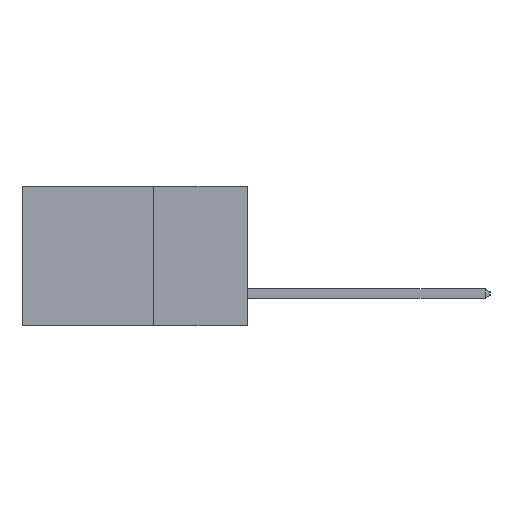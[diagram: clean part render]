
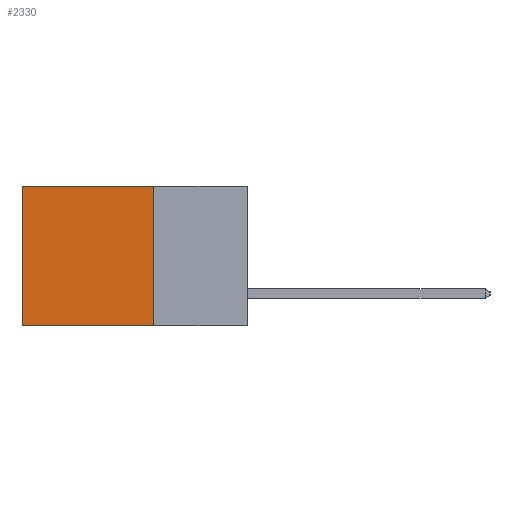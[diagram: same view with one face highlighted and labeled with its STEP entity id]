
A CAD part, left-side view. The second image highlights one B-rep face of the part: STEP entity #2330.
In plain terms, the highlighted planar face has unit normal (-1, 0, 0).
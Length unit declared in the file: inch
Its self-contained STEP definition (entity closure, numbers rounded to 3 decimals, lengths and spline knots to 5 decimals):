
#1316 = LINE ( 'NONE', #23785, #10888 ) ;
#2330 = ADVANCED_FACE ( 'NONE', ( #11259 ), #9148, .F. ) ;
#3410 = LINE ( 'NONE', #6248, #17305 ) ;
#4028 = CARTESIAN_POINT ( 'NONE',  ( 0.2615, 0.6, -0.37 ) ) ;
#4083 = DIRECTION ( 'NONE',  ( 0., 0., -1. ) ) ;
#4328 = VERTEX_POINT ( 'NONE', #19740 ) ;
#4990 = VERTEX_POINT ( 'NONE', #23582 ) ;
#5461 = VERTEX_POINT ( 'NONE', #18593 ) ;
#5703 = CARTESIAN_POINT ( 'NONE',  ( 0.2615, 0.25, -0.37 ) ) ;
#6026 = DIRECTION ( 'NONE',  ( 0., 0., -1. ) ) ;
#6052 = VECTOR ( 'NONE', #4083, 39.37008 ) ;
#6248 = CARTESIAN_POINT ( 'NONE',  ( 0.2615, 0.25, -0.37 ) ) ;
#6531 = EDGE_CURVE ( 'NONE', #5461, #8565, #3410, .T. ) ;
#8280 = DIRECTION ( 'NONE',  ( 0., 0., -1. ) ) ;
#8565 = VERTEX_POINT ( 'NONE', #13412 ) ;
#8781 = VECTOR ( 'NONE', #15842, 39.37008 ) ;
#9148 = PLANE ( 'NONE',  #9819 ) ;
#9819 = AXIS2_PLACEMENT_3D ( 'NONE', #5703, #10006, #8280 ) ;
#10006 = DIRECTION ( 'NONE',  ( 1., 0., 0. ) ) ;
#10357 = EDGE_CURVE ( 'NONE', #5461, #4328, #1316, .T. ) ;
#10888 = VECTOR ( 'NONE', #22719, 39.37008 ) ;
#11017 = ORIENTED_EDGE ( 'NONE', *, *, #10357, .T. ) ;
#11259 = FACE_OUTER_BOUND ( 'NONE', #14238, .T. ) ;
#12097 = CARTESIAN_POINT ( 'NONE',  ( 0.2615, 0.25, -0.37 ) ) ;
#12309 = LINE ( 'NONE', #4028, #6052 ) ;
#13412 = CARTESIAN_POINT ( 'NONE',  ( 0.2615, 0.25, -0.37 ) ) ;
#14238 = EDGE_LOOP ( 'NONE', ( #17604, #22334, #17381, #11017 ) ) ;
#14906 = EDGE_CURVE ( 'NONE', #4328, #4990, #12309, .T. ) ;
#15842 = DIRECTION ( 'NONE',  ( 0., 1., 0. ) ) ;
#17305 = VECTOR ( 'NONE', #6026, 39.37008 ) ;
#17381 = ORIENTED_EDGE ( 'NONE', *, *, #6531, .F. ) ;
#17604 = ORIENTED_EDGE ( 'NONE', *, *, #14906, .T. ) ;
#18593 = CARTESIAN_POINT ( 'NONE',  ( 0.2615, 0.25, 0. ) ) ;
#19740 = CARTESIAN_POINT ( 'NONE',  ( 0.2615, 0.6, 0. ) ) ;
#22334 = ORIENTED_EDGE ( 'NONE', *, *, #22765, .F. ) ;
#22719 = DIRECTION ( 'NONE',  ( 0., 1., 0. ) ) ;
#22765 = EDGE_CURVE ( 'NONE', #8565, #4990, #23549, .T. ) ;
#23549 = LINE ( 'NONE', #12097, #8781 ) ;
#23582 = CARTESIAN_POINT ( 'NONE',  ( 0.2615, 0.6, -0.37 ) ) ;
#23785 = CARTESIAN_POINT ( 'NONE',  ( 0.2615, 0.25, 0. ) ) ;
